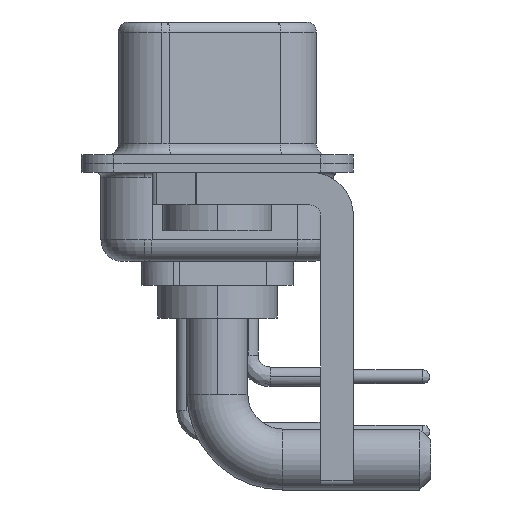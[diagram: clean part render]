
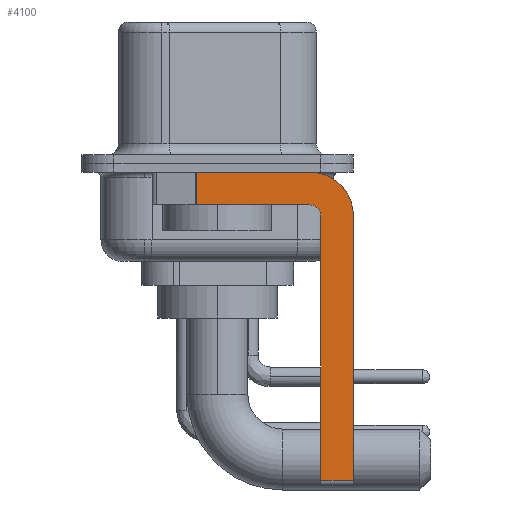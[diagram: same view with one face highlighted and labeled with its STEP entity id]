
A CAD part, left-side view. The second image highlights one B-rep face of the part: STEP entity #4100.
In plain terms, the highlighted planar face has unit normal (-1, 0, 0).
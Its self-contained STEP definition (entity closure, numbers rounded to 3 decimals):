
#363 = ORIENTED_EDGE ( 'NONE', *, *, #2964, .F. ) ;
#488 = DIRECTION ( 'NONE',  ( 0., 0., -1. ) ) ;
#665 = LINE ( 'NONE', #10712, #3266 ) ;
#742 = DIRECTION ( 'NONE',  ( 1., 0., 0. ) ) ;
#1077 = LINE ( 'NONE', #16785, #7630 ) ;
#2642 = CIRCLE ( 'NONE', #3448, 2. ) ;
#2644 = VERTEX_POINT ( 'NONE', #17613 ) ;
#2964 = EDGE_CURVE ( 'NONE', #2644, #12255, #18881, .T. ) ;
#3085 = VERTEX_POINT ( 'NONE', #21586 ) ;
#3266 = VECTOR ( 'NONE', #22678, 1000. ) ;
#3410 = CARTESIAN_POINT ( 'NONE',  ( -2.9, -4.75, -14.55 ) ) ;
#3448 = AXIS2_PLACEMENT_3D ( 'NONE', #16738, #5281, #14683 ) ;
#4100 = ADVANCED_FACE ( 'NONE', ( #6166 ), #14020, .F. ) ;
#4517 = VERTEX_POINT ( 'NONE', #21454 ) ;
#5068 = VERTEX_POINT ( 'NONE', #22824 ) ;
#5225 = LINE ( 'NONE', #24779, #25243 ) ;
#5281 = DIRECTION ( 'NONE',  ( 1., 0., 0. ) ) ;
#5461 = EDGE_CURVE ( 'NONE', #12255, #4517, #2642, .T. ) ;
#5829 = CARTESIAN_POINT ( 'NONE',  ( -2.9, -4.25, -1.9 ) ) ;
#5885 = CARTESIAN_POINT ( 'NONE',  ( -2.9, -4.25, -14.55 ) ) ;
#6018 = LINE ( 'NONE', #5885, #8573 ) ;
#6166 = FACE_OUTER_BOUND ( 'NONE', #17662, .T. ) ;
#6195 = ORIENTED_EDGE ( 'NONE', *, *, #5461, .F. ) ;
#6774 = EDGE_CURVE ( 'NONE', #2644, #3085, #5225, .T. ) ;
#7022 = DIRECTION ( 'NONE',  ( -1., 0., 0. ) ) ;
#7051 = CARTESIAN_POINT ( 'NONE',  ( -2.9, 3., -0.4 ) ) ;
#7379 = LINE ( 'NONE', #5829, #25450 ) ;
#7630 = VECTOR ( 'NONE', #9328, 1000. ) ;
#7905 = EDGE_CURVE ( 'NONE', #9111, #25221, #15497, .T. ) ;
#8481 = CARTESIAN_POINT ( 'NONE',  ( -2.9, -4.25, -2.4 ) ) ;
#8573 = VECTOR ( 'NONE', #13873, 1000. ) ;
#9103 = VECTOR ( 'NONE', #24301, 1000. ) ;
#9111 = VERTEX_POINT ( 'NONE', #12131 ) ;
#9206 = DIRECTION ( 'NONE',  ( 0., 0., 1. ) ) ;
#9328 = DIRECTION ( 'NONE',  ( 0., 0., 1. ) ) ;
#10427 = EDGE_CURVE ( 'NONE', #4517, #5068, #665, .T. ) ;
#10712 = CARTESIAN_POINT ( 'NONE',  ( -2.9, -6.25, -2.4 ) ) ;
#10855 = ORIENTED_EDGE ( 'NONE', *, *, #10427, .F. ) ;
#10969 = ORIENTED_EDGE ( 'NONE', *, *, #6774, .T. ) ;
#11460 = VERTEX_POINT ( 'NONE', #3410 ) ;
#12131 = CARTESIAN_POINT ( 'NONE',  ( -2.9, -4.75, -2.4 ) ) ;
#12255 = VERTEX_POINT ( 'NONE', #19527 ) ;
#13077 = DIRECTION ( 'NONE',  ( 0., 0., -1. ) ) ;
#13537 = EDGE_CURVE ( 'NONE', #11460, #5068, #6018, .T. ) ;
#13873 = DIRECTION ( 'NONE',  ( 0., -1., 0. ) ) ;
#14020 = PLANE ( 'NONE',  #24370 ) ;
#14354 = EDGE_CURVE ( 'NONE', #25221, #3085, #7379, .T. ) ;
#14683 = DIRECTION ( 'NONE',  ( 0., 0., -1. ) ) ;
#15497 = CIRCLE ( 'NONE', #25344, 0.5 ) ;
#15543 = ORIENTED_EDGE ( 'NONE', *, *, #13537, .T. ) ;
#16738 = CARTESIAN_POINT ( 'NONE',  ( -2.9, -4.25, -2.4 ) ) ;
#16785 = CARTESIAN_POINT ( 'NONE',  ( -2.9, -4.75, -14.8 ) ) ;
#17183 = ORIENTED_EDGE ( 'NONE', *, *, #7905, .F. ) ;
#17430 = CARTESIAN_POINT ( 'NONE',  ( -2.9, -4.25, -2.4 ) ) ;
#17613 = CARTESIAN_POINT ( 'NONE',  ( -2.9, 0.978, -0.4 ) ) ;
#17662 = EDGE_LOOP ( 'NONE', ( #363, #10969, #22359, #17183, #24179, #15543, #10855, #6195 ) ) ;
#18881 = LINE ( 'NONE', #7051, #9103 ) ;
#19527 = CARTESIAN_POINT ( 'NONE',  ( -2.9, -4.25, -0.4 ) ) ;
#19894 = CARTESIAN_POINT ( 'NONE',  ( -2.9, -4.25, -1.9 ) ) ;
#21454 = CARTESIAN_POINT ( 'NONE',  ( -2.9, -6.25, -2.4 ) ) ;
#21586 = CARTESIAN_POINT ( 'NONE',  ( -2.9, 0.978, -1.9 ) ) ;
#22359 = ORIENTED_EDGE ( 'NONE', *, *, #14354, .F. ) ;
#22678 = DIRECTION ( 'NONE',  ( 0., 0., -1. ) ) ;
#22824 = CARTESIAN_POINT ( 'NONE',  ( -2.9, -6.25, -14.55 ) ) ;
#23498 = EDGE_CURVE ( 'NONE', #11460, #9111, #1077, .T. ) ;
#24179 = ORIENTED_EDGE ( 'NONE', *, *, #23498, .F. ) ;
#24301 = DIRECTION ( 'NONE',  ( 0., -1., 0. ) ) ;
#24370 = AXIS2_PLACEMENT_3D ( 'NONE', #8481, #742, #488 ) ;
#24779 = CARTESIAN_POINT ( 'NONE',  ( -2.9, 0.978, -1.9 ) ) ;
#24999 = DIRECTION ( 'NONE',  ( 0., 1., 0. ) ) ;
#25221 = VERTEX_POINT ( 'NONE', #19894 ) ;
#25243 = VECTOR ( 'NONE', #13077, 1000. ) ;
#25344 = AXIS2_PLACEMENT_3D ( 'NONE', #17430, #7022, #9206 ) ;
#25450 = VECTOR ( 'NONE', #24999, 1000. ) ;
